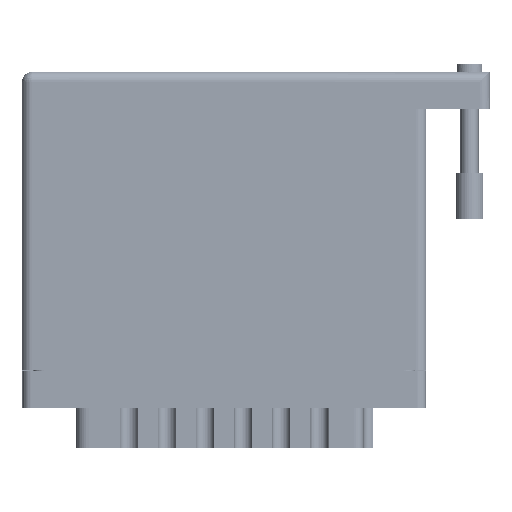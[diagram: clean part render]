
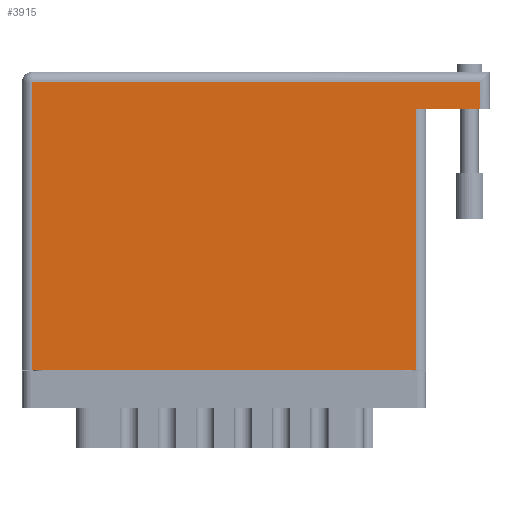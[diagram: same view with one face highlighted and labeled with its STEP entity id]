
A CAD part, front view. The second image highlights one B-rep face of the part: STEP entity #3915.
In plain terms, the highlighted face is planar.
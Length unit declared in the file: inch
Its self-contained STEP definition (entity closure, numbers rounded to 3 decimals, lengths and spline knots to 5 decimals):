
#682 = DIRECTION ( 'NONE',  ( -1., 0., 0. ) ) ;
#3089 = CARTESIAN_POINT ( 'NONE',  ( 0.07, 0., 0. ) ) ;
#3915 = ADVANCED_FACE ( 'NONE', ( #8978 ), #76290, .F. ) ;
#4734 = VERTEX_POINT ( 'NONE', #58980 ) ;
#8627 = VERTEX_POINT ( 'NONE', #55450 ) ;
#8978 = FACE_OUTER_BOUND ( 'NONE', #64338, .T. ) ;
#10058 = LINE ( 'NONE', #61742, #78699 ) ;
#15944 = LINE ( 'NONE', #45218, #63828 ) ;
#18766 = CARTESIAN_POINT ( 'NONE',  ( 2.685, 1.774, 0. ) ) ;
#19198 = VERTEX_POINT ( 'NONE', #18766 ) ;
#23912 = ORIENTED_EDGE ( 'NONE', *, *, #52821, .T. ) ;
#25093 = CARTESIAN_POINT ( 'NONE',  ( 3.12, 1.96, 0. ) ) ;
#25527 = CARTESIAN_POINT ( 'NONE',  ( 2.685, 0., 0. ) ) ;
#25950 = DIRECTION ( 'NONE',  ( 1., 0., 0. ) ) ;
#30749 = DIRECTION ( 'NONE',  ( 0., 1., 0. ) ) ;
#33110 = VERTEX_POINT ( 'NONE', #3089 ) ;
#34503 = VERTEX_POINT ( 'NONE', #25527 ) ;
#38229 = CARTESIAN_POINT ( 'NONE',  ( 0., 2.03, 0. ) ) ;
#40731 = CARTESIAN_POINT ( 'NONE',  ( 0.07, 0., 0. ) ) ;
#41037 = EDGE_CURVE ( 'NONE', #33110, #34503, #69371, .T. ) ;
#43716 = EDGE_CURVE ( 'NONE', #8627, #33110, #62656, .T. ) ;
#44879 = VERTEX_POINT ( 'NONE', #25093 ) ;
#44900 = VECTOR ( 'NONE', #54956, 39.37008 ) ;
#45218 = CARTESIAN_POINT ( 'NONE',  ( 0., 1.96, 0. ) ) ;
#48683 = ORIENTED_EDGE ( 'NONE', *, *, #76508, .T. ) ;
#51553 = ORIENTED_EDGE ( 'NONE', *, *, #60389, .F. ) ;
#52821 = EDGE_CURVE ( 'NONE', #4734, #44879, #60479, .T. ) ;
#54956 = DIRECTION ( 'NONE',  ( -1., 0., 0. ) ) ;
#55204 = CARTESIAN_POINT ( 'NONE',  ( 0., 0., 0. ) ) ;
#55450 = CARTESIAN_POINT ( 'NONE',  ( 0.07, 1.96, 0. ) ) ;
#57201 = EDGE_CURVE ( 'NONE', #34503, #19198, #10058, .T. ) ;
#57507 = ORIENTED_EDGE ( 'NONE', *, *, #57201, .T. ) ;
#57804 = ORIENTED_EDGE ( 'NONE', *, *, #41037, .T. ) ;
#58980 = CARTESIAN_POINT ( 'NONE',  ( 3.12, 1.774, 0. ) ) ;
#60389 = EDGE_CURVE ( 'NONE', #4734, #19198, #63226, .T. ) ;
#60479 = LINE ( 'NONE', #75624, #78118 ) ;
#61381 = AXIS2_PLACEMENT_3D ( 'NONE', #38229, #82654, #682 ) ;
#61742 = CARTESIAN_POINT ( 'NONE',  ( 2.685, 1.774, 0. ) ) ;
#62656 = LINE ( 'NONE', #40731, #92764 ) ;
#63226 = LINE ( 'NONE', #72016, #44900 ) ;
#63828 = VECTOR ( 'NONE', #69084, 39.37008 ) ;
#64338 = EDGE_LOOP ( 'NONE', ( #57804, #57507, #51553, #23912, #48683, #67775 ) ) ;
#67775 = ORIENTED_EDGE ( 'NONE', *, *, #43716, .T. ) ;
#69084 = DIRECTION ( 'NONE',  ( -1., 0., 0. ) ) ;
#69371 = LINE ( 'NONE', #55204, #71066 ) ;
#70479 = DIRECTION ( 'NONE',  ( 0., -1., 0. ) ) ;
#71066 = VECTOR ( 'NONE', #25950, 39.37008 ) ;
#72016 = CARTESIAN_POINT ( 'NONE',  ( 3.19, 1.774, 0. ) ) ;
#75624 = CARTESIAN_POINT ( 'NONE',  ( 3.12, 2.03, 0. ) ) ;
#76290 = PLANE ( 'NONE',  #61381 ) ;
#76508 = EDGE_CURVE ( 'NONE', #44879, #8627, #15944, .T. ) ;
#78118 = VECTOR ( 'NONE', #30749, 39.37008 ) ;
#78699 = VECTOR ( 'NONE', #84224, 39.37008 ) ;
#82654 = DIRECTION ( 'NONE',  ( 0., 0., -1. ) ) ;
#84224 = DIRECTION ( 'NONE',  ( 0., 1., 0. ) ) ;
#92764 = VECTOR ( 'NONE', #70479, 39.37008 ) ;
